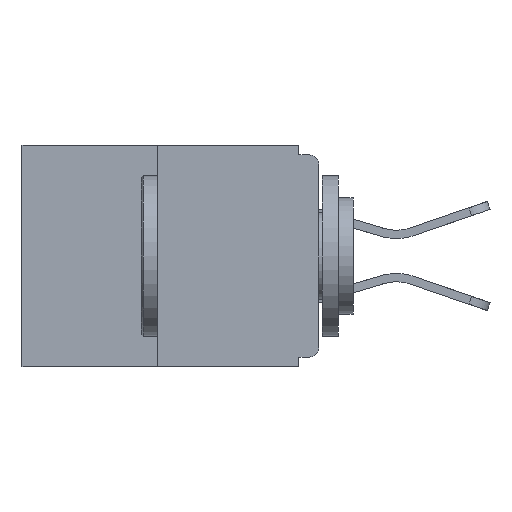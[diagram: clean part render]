
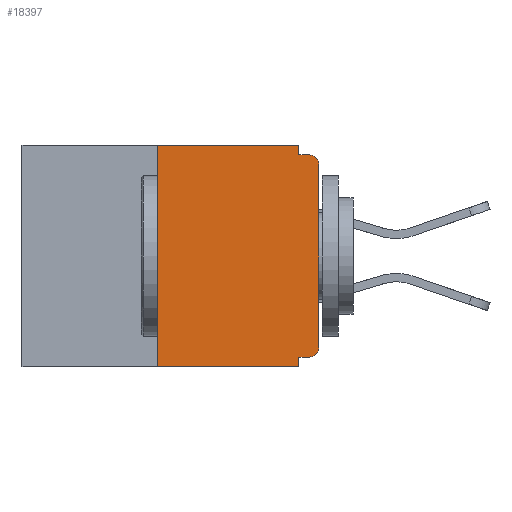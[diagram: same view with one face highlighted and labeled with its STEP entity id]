
A CAD part, left-side view. The second image highlights one B-rep face of the part: STEP entity #18397.
In plain terms, the highlighted planar face has unit normal (-1, 0, 0).
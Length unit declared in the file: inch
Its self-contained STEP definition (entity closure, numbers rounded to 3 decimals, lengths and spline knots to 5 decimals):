
#133 = CARTESIAN_POINT ( 'NONE',  ( 0., 0., -0.313 ) ) ;
#411 = VECTOR ( 'NONE', #15625, 39.37008 ) ;
#480 = LINE ( 'NONE', #8530, #26890 ) ;
#633 = DIRECTION ( 'NONE',  ( 1., 0., 0. ) ) ;
#724 = DIRECTION ( 'NONE',  ( 0., 0., -1. ) ) ;
#1307 = VECTOR ( 'NONE', #11170, 39.37008 ) ;
#1374 = LINE ( 'NONE', #12314, #2055 ) ;
#2008 = CARTESIAN_POINT ( 'NONE',  ( 0., 0.015, -0.313 ) ) ;
#2055 = VECTOR ( 'NONE', #24611, 39.37008 ) ;
#2094 = VERTEX_POINT ( 'NONE', #21951 ) ;
#2287 = AXIS2_PLACEMENT_3D ( 'NONE', #2008, #6192, #14764 ) ;
#2314 = EDGE_CURVE ( 'NONE', #6723, #18478, #9919, .T. ) ;
#2788 = VERTEX_POINT ( 'NONE', #24278 ) ;
#2859 = CARTESIAN_POINT ( 'NONE',  ( 0., 0.25, -0.343 ) ) ;
#2937 = EDGE_CURVE ( 'NONE', #2094, #2788, #20697, .T. ) ;
#3077 = VECTOR ( 'NONE', #16905, 39.37008 ) ;
#3160 = FACE_OUTER_BOUND ( 'NONE', #8014, .T. ) ;
#3181 = CIRCLE ( 'NONE', #19747, 0.015 ) ;
#3297 = CARTESIAN_POINT ( 'NONE',  ( 0., 0.031, -0.343 ) ) ;
#3368 = VECTOR ( 'NONE', #12854, 39.37008 ) ;
#3416 = CARTESIAN_POINT ( 'NONE',  ( 0., 0.25, 0. ) ) ;
#3787 = ORIENTED_EDGE ( 'NONE', *, *, #6826, .F. ) ;
#4471 = VERTEX_POINT ( 'NONE', #2859 ) ;
#4886 = CARTESIAN_POINT ( 'NONE',  ( 0., 0., -0.328 ) ) ;
#4976 = CARTESIAN_POINT ( 'NONE',  ( 0., 0.25, 0. ) ) ;
#5469 = CARTESIAN_POINT ( 'NONE',  ( 0., 0.031, 0. ) ) ;
#5924 = DIRECTION ( 'NONE',  ( -1., 0., 0. ) ) ;
#6192 = DIRECTION ( 'NONE',  ( -1., 0., 0. ) ) ;
#6242 = CARTESIAN_POINT ( 'NONE',  ( 0., 0.031, -0.343 ) ) ;
#6723 = VERTEX_POINT ( 'NONE', #25219 ) ;
#6826 = EDGE_CURVE ( 'NONE', #19112, #6723, #18643, .T. ) ;
#7320 = EDGE_CURVE ( 'NONE', #2094, #22042, #19261, .T. ) ;
#7331 = VERTEX_POINT ( 'NONE', #24978 ) ;
#7386 = ORIENTED_EDGE ( 'NONE', *, *, #2314, .F. ) ;
#7559 = ORIENTED_EDGE ( 'NONE', *, *, #7320, .T. ) ;
#8014 = EDGE_LOOP ( 'NONE', ( #16352, #22779, #10552, #10039, #25657, #7559, #14733, #24213, #7386, #3787 ) ) ;
#8094 = VECTOR ( 'NONE', #13430, 39.37008 ) ;
#8530 = CARTESIAN_POINT ( 'NONE',  ( 0., 0., 0. ) ) ;
#8836 = EDGE_CURVE ( 'NONE', #4471, #14732, #26991, .T. ) ;
#9919 = LINE ( 'NONE', #23291, #3077 ) ;
#10039 = ORIENTED_EDGE ( 'NONE', *, *, #15165, .F. ) ;
#10552 = ORIENTED_EDGE ( 'NONE', *, *, #24868, .T. ) ;
#11170 = DIRECTION ( 'NONE',  ( 0., 0., -1. ) ) ;
#11316 = CARTESIAN_POINT ( 'NONE',  ( 0., 0.46, -0.343 ) ) ;
#11379 = DIRECTION ( 'NONE',  ( 0., 0., 1. ) ) ;
#12314 = CARTESIAN_POINT ( 'NONE',  ( 0., 0.46, 0. ) ) ;
#12722 = AXIS2_PLACEMENT_3D ( 'NONE', #23350, #633, #724 ) ;
#12854 = DIRECTION ( 'NONE',  ( 0., 1., 0. ) ) ;
#13257 = EDGE_CURVE ( 'NONE', #22042, #7331, #480, .T. ) ;
#13430 = DIRECTION ( 'NONE',  ( 0., -1., 0. ) ) ;
#14241 = DIRECTION ( 'NONE',  ( 0., 0., -1. ) ) ;
#14732 = VERTEX_POINT ( 'NONE', #3416 ) ;
#14733 = ORIENTED_EDGE ( 'NONE', *, *, #13257, .T. ) ;
#14764 = DIRECTION ( 'NONE',  ( 0., 0., -1. ) ) ;
#15165 = EDGE_CURVE ( 'NONE', #2788, #20007, #23281, .T. ) ;
#15269 = CARTESIAN_POINT ( 'NONE',  ( 0., 0.031, 0. ) ) ;
#15321 = EDGE_CURVE ( 'NONE', #14732, #19112, #1374, .T. ) ;
#15625 = DIRECTION ( 'NONE',  ( 0., 0., -1. ) ) ;
#16352 = ORIENTED_EDGE ( 'NONE', *, *, #15321, .F. ) ;
#16905 = DIRECTION ( 'NONE',  ( 0., -1., 0. ) ) ;
#18397 = ADVANCED_FACE ( 'NONE', ( #3160 ), #25703, .F. ) ;
#18478 = VERTEX_POINT ( 'NONE', #26224 ) ;
#18643 = LINE ( 'NONE', #15269, #1307 ) ;
#18767 = DIRECTION ( 'NONE',  ( 0., 0., 1. ) ) ;
#19112 = VERTEX_POINT ( 'NONE', #5469 ) ;
#19261 = CIRCLE ( 'NONE', #2287, 0.015 ) ;
#19747 = AXIS2_PLACEMENT_3D ( 'NONE', #26694, #5924, #14241 ) ;
#20007 = VERTEX_POINT ( 'NONE', #6242 ) ;
#20697 = LINE ( 'NONE', #4886, #3368 ) ;
#20782 = EDGE_CURVE ( 'NONE', #7331, #18478, #3181, .T. ) ;
#21951 = CARTESIAN_POINT ( 'NONE',  ( 0., 0.015, -0.328 ) ) ;
#22042 = VERTEX_POINT ( 'NONE', #133 ) ;
#22779 = ORIENTED_EDGE ( 'NONE', *, *, #8836, .F. ) ;
#23281 = LINE ( 'NONE', #3297, #411 ) ;
#23291 = CARTESIAN_POINT ( 'NONE',  ( 0., 0., -0.015 ) ) ;
#23350 = CARTESIAN_POINT ( 'NONE',  ( 0., 0.46, 0. ) ) ;
#23749 = VECTOR ( 'NONE', #11379, 39.37008 ) ;
#24213 = ORIENTED_EDGE ( 'NONE', *, *, #20782, .T. ) ;
#24278 = CARTESIAN_POINT ( 'NONE',  ( 0., 0.031, -0.328 ) ) ;
#24611 = DIRECTION ( 'NONE',  ( 0., -1., 0. ) ) ;
#24868 = EDGE_CURVE ( 'NONE', #4471, #20007, #26028, .T. ) ;
#24978 = CARTESIAN_POINT ( 'NONE',  ( 0., 0., -0.03 ) ) ;
#25219 = CARTESIAN_POINT ( 'NONE',  ( 0., 0.031, -0.015 ) ) ;
#25657 = ORIENTED_EDGE ( 'NONE', *, *, #2937, .F. ) ;
#25703 = PLANE ( 'NONE',  #12722 ) ;
#26028 = LINE ( 'NONE', #11316, #8094 ) ;
#26224 = CARTESIAN_POINT ( 'NONE',  ( 0., 0.015, -0.015 ) ) ;
#26694 = CARTESIAN_POINT ( 'NONE',  ( 0., 0.015, -0.03 ) ) ;
#26890 = VECTOR ( 'NONE', #18767, 39.37008 ) ;
#26991 = LINE ( 'NONE', #4976, #23749 ) ;
